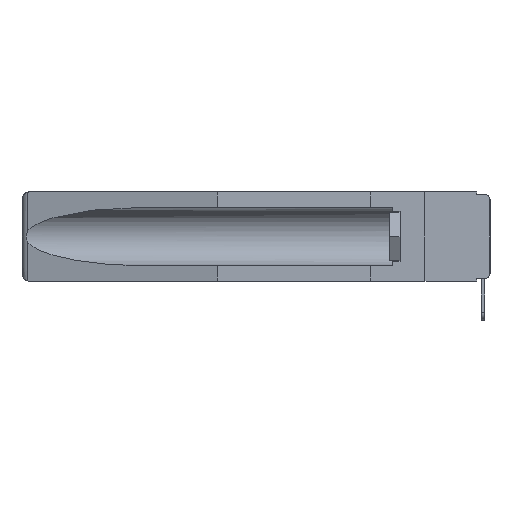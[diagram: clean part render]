
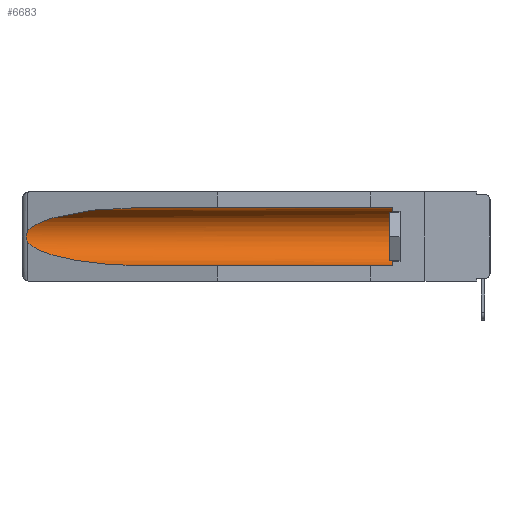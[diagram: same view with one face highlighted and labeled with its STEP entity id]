
A CAD part, left-side view. The second image highlights one B-rep face of the part: STEP entity #6683.
In plain terms, the highlighted cylindrical face has radius 2.857 mm (diameter 5.715 mm), a partial arc.
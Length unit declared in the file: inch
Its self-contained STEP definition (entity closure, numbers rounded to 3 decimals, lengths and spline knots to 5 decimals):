
#150 = CARTESIAN_POINT ( 'NONE',  ( 0.155, 0.126, -0.059 ) ) ;
#239 = CARTESIAN_POINT ( 'NONE',  ( 0.21114, 1.30732, -0.059 ) ) ;
#452 = EDGE_CURVE ( 'NONE', #8977, #16624, #6833, .T. ) ;
#834 = CARTESIAN_POINT ( 'NONE',  ( 0.26537, 1.52718, -0.19328 ) ) ;
#1037 = VERTEX_POINT ( 'NONE', #5456 ) ;
#1357 = DIRECTION ( 'NONE',  ( 0., 0., 1. ) ) ;
#1594 = ORIENTED_EDGE ( 'NONE', *, *, #6442, .T. ) ;
#2296 = VERTEX_POINT ( 'NONE', #5506 ) ;
#3246 = CARTESIAN_POINT ( 'NONE',  ( 0.26597, 1.52961, -0.15275 ) ) ;
#3306 = CARTESIAN_POINT ( 'NONE',  ( 0.26537, 1.52718, -0.19328 ) ) ;
#3403 = VECTOR ( 'NONE', #12283, 39.37008 ) ;
#4197 = VECTOR ( 'NONE', #14822, 39.37008 ) ;
#4376 = ORIENTED_EDGE ( 'NONE', *, *, #15060, .T. ) ;
#4722 = CARTESIAN_POINT ( 'NONE',  ( 0.26654, 1.53092, -0.15636 ) ) ;
#5130 = CARTESIAN_POINT ( 'NONE',  ( 0.155, -0.30754, -0.1715 ) ) ;
#5456 = CARTESIAN_POINT ( 'NONE',  ( 0.155, 1.07973, -0.284 ) ) ;
#5502 = B_SPLINE_CURVE_WITH_KNOTS ( 'NONE', 3,
 ( #10981, #3246, #4722, #12293, #13756, #12516, #16151, #15091, #6041, #3306 ),
 .UNSPECIFIED., .F., .F.,
 ( 4, 2, 2, 2, 4 ),
 ( 0., 0.00029, 0.00058, 0.00087, 0.00117 ),
 .UNSPECIFIED. ) ;
#5506 = CARTESIAN_POINT ( 'NONE',  ( 0.155, 0.126, -0.284 ) ) ;
#5626 = LINE ( 'NONE', #5855, #3403 ) ;
#5855 = CARTESIAN_POINT ( 'NONE',  ( 0.155, -0.30754, -0.284 ) ) ;
#5944 = CARTESIAN_POINT ( 'NONE',  ( 0.155, 1.07973, -0.284 ) ) ;
#6018 = EDGE_CURVE ( 'NONE', #13905, #8809, #5502, .T. ) ;
#6041 = CARTESIAN_POINT ( 'NONE',  ( 0.26597, 1.5296, -0.19026 ) ) ;
#6442 = EDGE_CURVE ( 'NONE', #8809, #1037, #10468, .T. ) ;
#6503 = DIRECTION ( 'NONE',  ( 0., 1., 0. ) ) ;
#6683 = ADVANCED_FACE ( 'NONE', ( #16660 ), #13257, .F. ) ;
#6833 = LINE ( 'NONE', #16109, #4197 ) ;
#6991 = ORIENTED_EDGE ( 'NONE', *, *, #452, .T. ) ;
#7509 = CARTESIAN_POINT ( 'NONE',  ( 0.26537, 1.52718, -0.14972 ) ) ;
#8571 = CARTESIAN_POINT ( 'NONE',  ( 0.21114, 1.30732, -0.284 ) ) ;
#8733 = ORIENTED_EDGE ( 'NONE', *, *, #11708, .T. ) ;
#8809 = VERTEX_POINT ( 'NONE', #11559 ) ;
#8977 = VERTEX_POINT ( 'NONE', #150 ) ;
#9059 = DIRECTION ( 'NONE',  ( 0., -1., 0. ) ) ;
#9509 = CIRCLE ( 'NONE', #16578, 0.1125 ) ;
#10468 =( BOUNDED_CURVE ( )  B_SPLINE_CURVE ( 3, ( #834, #12435, #8571, #5944 ),
 .UNSPECIFIED., .F., .T. ) 
 B_SPLINE_CURVE_WITH_KNOTS ( ( 4, 4 ),
 ( 0.1948, 1.5708 ),
 .UNSPECIFIED. ) 
 CURVE ( )  GEOMETRIC_REPRESENTATION_ITEM ( )  RATIONAL_B_SPLINE_CURVE ( ( 1., 0.848, 0.848, 1. ) ) 
 REPRESENTATION_ITEM ( '' )  );
#10771 =( BOUNDED_CURVE ( )  B_SPLINE_CURVE ( 3, ( #13109, #239, #11867, #7509 ),
 .UNSPECIFIED., .F., .F. ) 
 B_SPLINE_CURVE_WITH_KNOTS ( ( 4, 4 ),
 ( 4.71239, 6.08839 ),
 .UNSPECIFIED. ) 
 CURVE ( )  GEOMETRIC_REPRESENTATION_ITEM ( )  RATIONAL_B_SPLINE_CURVE ( ( 1., 0.848, 0.848, 1. ) ) 
 REPRESENTATION_ITEM ( '' )  );
#10981 = CARTESIAN_POINT ( 'NONE',  ( 0.26537, 1.52718, -0.14972 ) ) ;
#11129 = AXIS2_PLACEMENT_3D ( 'NONE', #5130, #6503, #15497 ) ;
#11559 = CARTESIAN_POINT ( 'NONE',  ( 0.26537, 1.52718, -0.19328 ) ) ;
#11663 = CARTESIAN_POINT ( 'NONE',  ( 0.155, 0.126, -0.1715 ) ) ;
#11708 = EDGE_CURVE ( 'NONE', #2296, #8977, #9509, .T. ) ;
#11785 = ORIENTED_EDGE ( 'NONE', *, *, #6018, .T. ) ;
#11867 = CARTESIAN_POINT ( 'NONE',  ( 0.25451, 1.48313, -0.09465 ) ) ;
#11877 = EDGE_LOOP ( 'NONE', ( #4376, #11785, #1594, #12781, #8733, #6991 ) ) ;
#12283 = DIRECTION ( 'NONE',  ( 0., 1., 0. ) ) ;
#12293 = CARTESIAN_POINT ( 'NONE',  ( 0.2673, 1.5327, -0.16383 ) ) ;
#12435 = CARTESIAN_POINT ( 'NONE',  ( 0.25451, 1.48313, -0.24835 ) ) ;
#12508 = CARTESIAN_POINT ( 'NONE',  ( 0.26537, 1.52718, -0.14972 ) ) ;
#12516 = CARTESIAN_POINT ( 'NONE',  ( 0.2675, 1.53308, -0.17534 ) ) ;
#12781 = ORIENTED_EDGE ( 'NONE', *, *, #14836, .F. ) ;
#13109 = CARTESIAN_POINT ( 'NONE',  ( 0.155, 1.07973, -0.059 ) ) ;
#13257 = CYLINDRICAL_SURFACE ( 'NONE', #11129, 0.1125 ) ;
#13756 = CARTESIAN_POINT ( 'NONE',  ( 0.2675, 1.53308, -0.16763 ) ) ;
#13905 = VERTEX_POINT ( 'NONE', #12508 ) ;
#14804 = CARTESIAN_POINT ( 'NONE',  ( 0.155, 1.07973, -0.059 ) ) ;
#14822 = DIRECTION ( 'NONE',  ( 0., 1., 0. ) ) ;
#14836 = EDGE_CURVE ( 'NONE', #2296, #1037, #5626, .T. ) ;
#15060 = EDGE_CURVE ( 'NONE', #16624, #13905, #10771, .T. ) ;
#15091 = CARTESIAN_POINT ( 'NONE',  ( 0.26655, 1.53094, -0.18657 ) ) ;
#15497 = DIRECTION ( 'NONE',  ( 0., 0., 1. ) ) ;
#16109 = CARTESIAN_POINT ( 'NONE',  ( 0.155, -0.30754, -0.059 ) ) ;
#16151 = CARTESIAN_POINT ( 'NONE',  ( 0.2673, 1.53269, -0.17917 ) ) ;
#16578 = AXIS2_PLACEMENT_3D ( 'NONE', #11663, #9059, #1357 ) ;
#16624 = VERTEX_POINT ( 'NONE', #14804 ) ;
#16660 = FACE_OUTER_BOUND ( 'NONE', #11877, .T. ) ;
